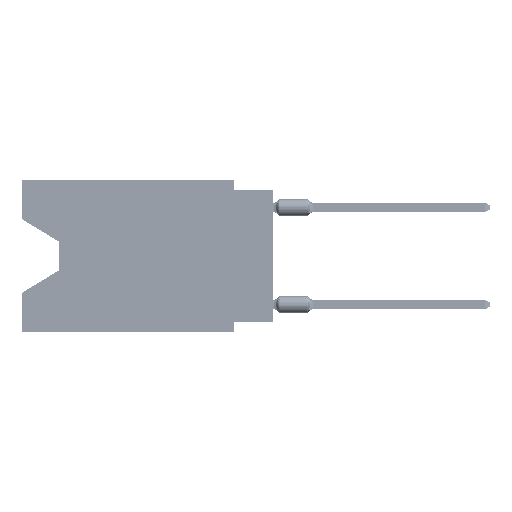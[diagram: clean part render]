
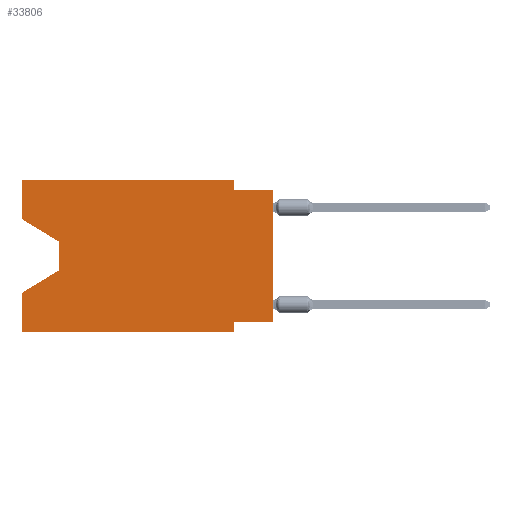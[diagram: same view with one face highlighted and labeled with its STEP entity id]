
A CAD part, left-side view. The second image highlights one B-rep face of the part: STEP entity #33806.
In plain terms, the highlighted planar face has unit normal (-1, 0, 0).
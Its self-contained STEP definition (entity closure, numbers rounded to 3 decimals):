
#212 = DIRECTION ( 'NONE',  ( 0., 0., 1. ) ) ;
#2128 = VERTEX_POINT ( 'NONE', #60131 ) ;
#2181 = CARTESIAN_POINT ( 'NONE',  ( 0., 0., -9.271 ) ) ;
#3387 = PLANE ( 'NONE',  #27570 ) ;
#3514 = LINE ( 'NONE', #31317, #35722 ) ;
#4176 = EDGE_CURVE ( 'NONE', #27108, #15293, #34705, .T. ) ;
#6121 = VECTOR ( 'NONE', #38676, 1000. ) ;
#6468 = ORIENTED_EDGE ( 'NONE', *, *, #44030, .F. ) ;
#6730 = DIRECTION ( 'NONE',  ( 0., 0., -1. ) ) ;
#8015 = VERTEX_POINT ( 'NONE', #47642 ) ;
#9387 = ORIENTED_EDGE ( 'NONE', *, *, #23576, .T. ) ;
#9863 = CARTESIAN_POINT ( 'NONE',  ( 0., 16.383, 0. ) ) ;
#10095 = DIRECTION ( 'NONE',  ( 0., 1., 0. ) ) ;
#10221 = FACE_OUTER_BOUND ( 'NONE', #56430, .T. ) ;
#10262 = CARTESIAN_POINT ( 'NONE',  ( 0., 16.383, -9.906 ) ) ;
#10333 = ORIENTED_EDGE ( 'NONE', *, *, #53024, .T. ) ;
#11802 = CARTESIAN_POINT ( 'NONE',  ( 0., 16.383, 0. ) ) ;
#12404 = DIRECTION ( 'NONE',  ( 0., 0., -1. ) ) ;
#12428 = ORIENTED_EDGE ( 'NONE', *, *, #16042, .F. ) ;
#15293 = VERTEX_POINT ( 'NONE', #17139 ) ;
#16042 = EDGE_CURVE ( 'NONE', #54283, #8015, #69364, .T. ) ;
#16806 = EDGE_CURVE ( 'NONE', #53462, #2128, #20410, .T. ) ;
#17079 = VECTOR ( 'NONE', #12404, 1000. ) ;
#17139 = CARTESIAN_POINT ( 'NONE',  ( 0., 2.54, -0.635 ) ) ;
#19116 = CARTESIAN_POINT ( 'NONE',  ( 0., 16.383, -2.546 ) ) ;
#19563 = LINE ( 'NONE', #19116, #76976 ) ;
#20309 = VERTEX_POINT ( 'NONE', #82006 ) ;
#20410 = LINE ( 'NONE', #48206, #67727 ) ;
#21613 = LINE ( 'NONE', #69473, #70927 ) ;
#22188 = VECTOR ( 'NONE', #50444, 1000. ) ;
#23576 = EDGE_CURVE ( 'NONE', #20309, #53462, #19563, .T. ) ;
#23611 = VECTOR ( 'NONE', #76127, 1000. ) ;
#23881 = DIRECTION ( 'NONE',  ( 1., 0., 0. ) ) ;
#25234 = EDGE_CURVE ( 'NONE', #49504, #77739, #34639, .T. ) ;
#25833 = ORIENTED_EDGE ( 'NONE', *, *, #16806, .T. ) ;
#26492 = CARTESIAN_POINT ( 'NONE',  ( 0., 13.97, -4.013 ) ) ;
#27108 = VERTEX_POINT ( 'NONE', #74588 ) ;
#27570 = AXIS2_PLACEMENT_3D ( 'NONE', #86317, #23881, #59425 ) ;
#31147 = ORIENTED_EDGE ( 'NONE', *, *, #85084, .F. ) ;
#31317 = CARTESIAN_POINT ( 'NONE',  ( 0., 0., 0. ) ) ;
#32220 = CARTESIAN_POINT ( 'NONE',  ( 0., 13.97, -5.893 ) ) ;
#32681 = LINE ( 'NONE', #46830, #54149 ) ;
#32900 = ORIENTED_EDGE ( 'NONE', *, *, #75346, .F. ) ;
#33688 = ORIENTED_EDGE ( 'NONE', *, *, #69691, .F. ) ;
#33806 = ADVANCED_FACE ( 'NONE', ( #10221 ), #3387, .F. ) ;
#34639 = LINE ( 'NONE', #76561, #23611 ) ;
#34705 = LINE ( 'NONE', #68893, #17079 ) ;
#35026 = DIRECTION ( 'NONE',  ( 0., -0.855, -0.519 ) ) ;
#35121 = CARTESIAN_POINT ( 'NONE',  ( 0., 2.54, -9.906 ) ) ;
#35722 = VECTOR ( 'NONE', #59104, 1000. ) ;
#38676 = DIRECTION ( 'NONE',  ( 0., -1., 0. ) ) ;
#39357 = EDGE_CURVE ( 'NONE', #54283, #50763, #3514, .T. ) ;
#39496 = DIRECTION ( 'NONE',  ( 0., 0.855, -0.519 ) ) ;
#41798 = EDGE_CURVE ( 'NONE', #49504, #89802, #21613, .T. ) ;
#43157 = CARTESIAN_POINT ( 'NONE',  ( 0., 0., -0.635 ) ) ;
#44030 = EDGE_CURVE ( 'NONE', #20309, #82110, #73314, .T. ) ;
#45208 = ORIENTED_EDGE ( 'NONE', *, *, #39357, .T. ) ;
#46830 = CARTESIAN_POINT ( 'NONE',  ( 0., 2.54, -9.906 ) ) ;
#47268 = DIRECTION ( 'NONE',  ( 0., 0., -1. ) ) ;
#47642 = CARTESIAN_POINT ( 'NONE',  ( 0., 2.54, -9.271 ) ) ;
#48206 = CARTESIAN_POINT ( 'NONE',  ( 0., 13.97, -4.013 ) ) ;
#49504 = VERTEX_POINT ( 'NONE', #10262 ) ;
#50444 = DIRECTION ( 'NONE',  ( 0., -1., 0. ) ) ;
#50763 = VERTEX_POINT ( 'NONE', #85935 ) ;
#53024 = EDGE_CURVE ( 'NONE', #2128, #89802, #78290, .T. ) ;
#53462 = VERTEX_POINT ( 'NONE', #26492 ) ;
#54149 = VECTOR ( 'NONE', #47268, 1000. ) ;
#54283 = VERTEX_POINT ( 'NONE', #2181 ) ;
#55700 = CARTESIAN_POINT ( 'NONE',  ( 0., 0., -9.271 ) ) ;
#56430 = EDGE_LOOP ( 'NONE', ( #9387, #25833, #10333, #76475, #70150, #32900, #12428, #45208, #33688, #81578, #31147, #6468 ) ) ;
#57727 = LINE ( 'NONE', #43157, #22188 ) ;
#58291 = CARTESIAN_POINT ( 'NONE',  ( 0., 16.383, 0. ) ) ;
#59104 = DIRECTION ( 'NONE',  ( 0., 0., 1. ) ) ;
#59425 = DIRECTION ( 'NONE',  ( 0., 0., -1. ) ) ;
#59658 = VECTOR ( 'NONE', #71971, 1000. ) ;
#60131 = CARTESIAN_POINT ( 'NONE',  ( 0., 13.97, -5.893 ) ) ;
#62579 = CARTESIAN_POINT ( 'NONE',  ( 0., 16.383, -7.36 ) ) ;
#67727 = VECTOR ( 'NONE', #6730, 1000. ) ;
#68893 = CARTESIAN_POINT ( 'NONE',  ( 0., 2.54, 0. ) ) ;
#69364 = LINE ( 'NONE', #55700, #85302 ) ;
#69473 = CARTESIAN_POINT ( 'NONE',  ( 0., 16.383, 0. ) ) ;
#69691 = EDGE_CURVE ( 'NONE', #15293, #50763, #57727, .T. ) ;
#70150 = ORIENTED_EDGE ( 'NONE', *, *, #25234, .T. ) ;
#70927 = VECTOR ( 'NONE', #212, 1000. ) ;
#71971 = DIRECTION ( 'NONE',  ( 0., 0., 1. ) ) ;
#73314 = LINE ( 'NONE', #58291, #59658 ) ;
#74588 = CARTESIAN_POINT ( 'NONE',  ( 0., 2.54, 0. ) ) ;
#75346 = EDGE_CURVE ( 'NONE', #8015, #77739, #32681, .T. ) ;
#76127 = DIRECTION ( 'NONE',  ( 0., -1., 0. ) ) ;
#76475 = ORIENTED_EDGE ( 'NONE', *, *, #41798, .F. ) ;
#76561 = CARTESIAN_POINT ( 'NONE',  ( 0., 16.383, -9.906 ) ) ;
#76976 = VECTOR ( 'NONE', #35026, 1000. ) ;
#77739 = VERTEX_POINT ( 'NONE', #35121 ) ;
#78290 = LINE ( 'NONE', #32220, #79890 ) ;
#79706 = LINE ( 'NONE', #11802, #6121 ) ;
#79890 = VECTOR ( 'NONE', #39496, 1000. ) ;
#81578 = ORIENTED_EDGE ( 'NONE', *, *, #4176, .F. ) ;
#82006 = CARTESIAN_POINT ( 'NONE',  ( 0., 16.383, -2.546 ) ) ;
#82110 = VERTEX_POINT ( 'NONE', #9863 ) ;
#85084 = EDGE_CURVE ( 'NONE', #82110, #27108, #79706, .T. ) ;
#85302 = VECTOR ( 'NONE', #10095, 1000. ) ;
#85935 = CARTESIAN_POINT ( 'NONE',  ( 0., 0., -0.635 ) ) ;
#86317 = CARTESIAN_POINT ( 'NONE',  ( 0., 16.383, 0. ) ) ;
#89802 = VERTEX_POINT ( 'NONE', #62579 ) ;
